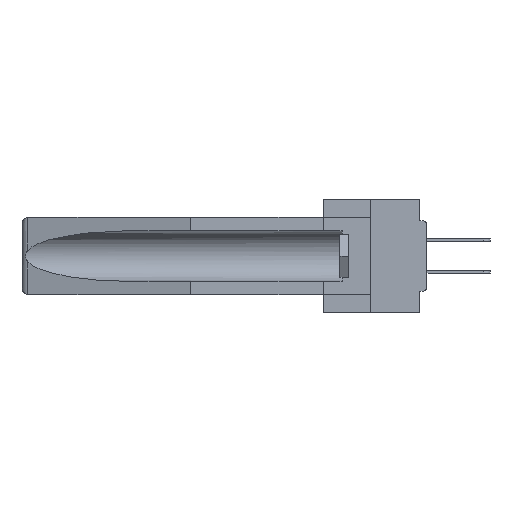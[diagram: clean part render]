
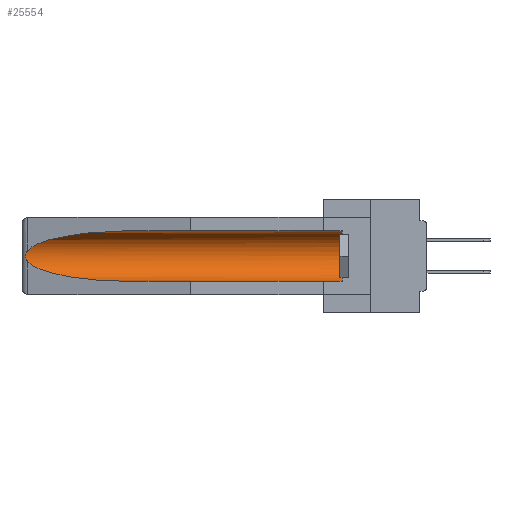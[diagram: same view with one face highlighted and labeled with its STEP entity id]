
A CAD part, left-side view. The second image highlights one B-rep face of the part: STEP entity #25554.
In plain terms, the highlighted cylindrical face has radius 2.857 mm (diameter 5.715 mm), a partial arc.
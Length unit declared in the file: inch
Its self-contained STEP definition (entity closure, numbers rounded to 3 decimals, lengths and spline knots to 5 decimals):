
#349 = EDGE_CURVE ( 'NONE', #12843, #17895, #983, .T. ) ;
#506 = VERTEX_POINT ( 'NONE', #14786 ) ;
#983 =( BOUNDED_CURVE ( )  B_SPLINE_CURVE ( 3, ( #24447, #27246, #11314, #16499 ),
 .UNSPECIFIED., .F., .F. ) 
 B_SPLINE_CURVE_WITH_KNOTS ( ( 4, 4 ),
 ( 4.71239, 6.08839 ),
 .UNSPECIFIED. ) 
 CURVE ( )  GEOMETRIC_REPRESENTATION_ITEM ( )  RATIONAL_B_SPLINE_CURVE ( ( 1., 0.848, 0.848, 1. ) ) 
 REPRESENTATION_ITEM ( '' )  );
#1634 = VECTOR ( 'NONE', #4664, 39.37008 ) ;
#1759 = AXIS2_PLACEMENT_3D ( 'NONE', #3451, #17104, #19829 ) ;
#2175 = CIRCLE ( 'NONE', #19865, 0.1125 ) ;
#3451 = CARTESIAN_POINT ( 'NONE',  ( 0.155, -0.30754, -0.1715 ) ) ;
#3897 = VECTOR ( 'NONE', #30911, 39.37008 ) ;
#4554 = CARTESIAN_POINT ( 'NONE',  ( 0.155, -0.30754, -0.284 ) ) ;
#4664 = DIRECTION ( 'NONE',  ( 0., 1., 0. ) ) ;
#4744 = DIRECTION ( 'NONE',  ( 0., 0., 1. ) ) ;
#4749 = VERTEX_POINT ( 'NONE', #17183 ) ;
#5481 = CARTESIAN_POINT ( 'NONE',  ( 0.21114, 1.30732, -0.284 ) ) ;
#5918 = ORIENTED_EDGE ( 'NONE', *, *, #8402, .T. ) ;
#6182 = CARTESIAN_POINT ( 'NONE',  ( 0.2673, 1.5327, -0.16383 ) ) ;
#6440 = CARTESIAN_POINT ( 'NONE',  ( 0.26597, 1.5296, -0.19026 ) ) ;
#8402 = EDGE_CURVE ( 'NONE', #28125, #16788, #17603, .T. ) ;
#8495 = CARTESIAN_POINT ( 'NONE',  ( 0.26537, 1.52718, -0.19328 ) ) ;
#9487 = CARTESIAN_POINT ( 'NONE',  ( 0.26537, 1.52718, -0.19328 ) ) ;
#11211 = CARTESIAN_POINT ( 'NONE',  ( 0.2675, 1.53308, -0.16763 ) ) ;
#11274 = ORIENTED_EDGE ( 'NONE', *, *, #27822, .T. ) ;
#11314 = CARTESIAN_POINT ( 'NONE',  ( 0.25451, 1.48313, -0.09465 ) ) ;
#11803 = EDGE_CURVE ( 'NONE', #506, #16788, #28668, .T. ) ;
#11893 = B_SPLINE_CURVE_WITH_KNOTS ( 'NONE', 3,
 ( #27144, #13857, #22145, #6182, #11211, #14679, #19572, #33063, #6440, #27606 ),
 .UNSPECIFIED., .F., .F.,
 ( 4, 2, 2, 2, 4 ),
 ( 0., 0.00029, 0.00058, 0.00087, 0.00117 ),
 .UNSPECIFIED. ) ;
#12843 = VERTEX_POINT ( 'NONE', #13403 ) ;
#13199 = ORIENTED_EDGE ( 'NONE', *, *, #349, .T. ) ;
#13403 = CARTESIAN_POINT ( 'NONE',  ( 0.155, 1.07973, -0.059 ) ) ;
#13857 = CARTESIAN_POINT ( 'NONE',  ( 0.26597, 1.52961, -0.15275 ) ) ;
#13952 = CARTESIAN_POINT ( 'NONE',  ( 0.25451, 1.48313, -0.24835 ) ) ;
#14679 = CARTESIAN_POINT ( 'NONE',  ( 0.2675, 1.53308, -0.17534 ) ) ;
#14732 = ORIENTED_EDGE ( 'NONE', *, *, #21017, .T. ) ;
#14786 = CARTESIAN_POINT ( 'NONE',  ( 0.155, 0.126, -0.284 ) ) ;
#15538 = CARTESIAN_POINT ( 'NONE',  ( 0.155, 0.126, -0.1715 ) ) ;
#16072 = CARTESIAN_POINT ( 'NONE',  ( 0.26537, 1.52718, -0.14972 ) ) ;
#16499 = CARTESIAN_POINT ( 'NONE',  ( 0.26537, 1.52718, -0.14972 ) ) ;
#16788 = VERTEX_POINT ( 'NONE', #32964 ) ;
#17104 = DIRECTION ( 'NONE',  ( 0., 1., 0. ) ) ;
#17183 = CARTESIAN_POINT ( 'NONE',  ( 0.155, 0.126, -0.059 ) ) ;
#17603 =( BOUNDED_CURVE ( )  B_SPLINE_CURVE ( 3, ( #8495, #13952, #5481, #26779 ),
 .UNSPECIFIED., .F., .F. ) 
 B_SPLINE_CURVE_WITH_KNOTS ( ( 4, 4 ),
 ( 0.1948, 1.5708 ),
 .UNSPECIFIED. ) 
 CURVE ( )  GEOMETRIC_REPRESENTATION_ITEM ( )  RATIONAL_B_SPLINE_CURVE ( ( 1., 0.848, 0.848, 1. ) ) 
 REPRESENTATION_ITEM ( '' )  );
#17895 = VERTEX_POINT ( 'NONE', #16072 ) ;
#19572 = CARTESIAN_POINT ( 'NONE',  ( 0.2673, 1.53269, -0.17917 ) ) ;
#19829 = DIRECTION ( 'NONE',  ( 0., 0., 1. ) ) ;
#19865 = AXIS2_PLACEMENT_3D ( 'NONE', #15538, #31248, #4744 ) ;
#21017 = EDGE_CURVE ( 'NONE', #17895, #28125, #11893, .T. ) ;
#22145 = CARTESIAN_POINT ( 'NONE',  ( 0.26654, 1.53092, -0.15636 ) ) ;
#22932 = CARTESIAN_POINT ( 'NONE',  ( 0.155, -0.30754, -0.059 ) ) ;
#24447 = CARTESIAN_POINT ( 'NONE',  ( 0.155, 1.07973, -0.059 ) ) ;
#25554 = ADVANCED_FACE ( 'NONE', ( #28925 ), #28104, .F. ) ;
#25887 = ORIENTED_EDGE ( 'NONE', *, *, #11803, .F. ) ;
#26641 = ORIENTED_EDGE ( 'NONE', *, *, #33832, .T. ) ;
#26779 = CARTESIAN_POINT ( 'NONE',  ( 0.155, 1.07973, -0.284 ) ) ;
#27144 = CARTESIAN_POINT ( 'NONE',  ( 0.26537, 1.52718, -0.14972 ) ) ;
#27246 = CARTESIAN_POINT ( 'NONE',  ( 0.21114, 1.30732, -0.059 ) ) ;
#27606 = CARTESIAN_POINT ( 'NONE',  ( 0.26537, 1.52718, -0.19328 ) ) ;
#27822 = EDGE_CURVE ( 'NONE', #506, #4749, #2175, .T. ) ;
#28104 = CYLINDRICAL_SURFACE ( 'NONE', #1759, 0.1125 ) ;
#28125 = VERTEX_POINT ( 'NONE', #9487 ) ;
#28668 = LINE ( 'NONE', #4554, #1634 ) ;
#28925 = FACE_OUTER_BOUND ( 'NONE', #30764, .T. ) ;
#30764 = EDGE_LOOP ( 'NONE', ( #13199, #14732, #5918, #25887, #11274, #26641 ) ) ;
#30911 = DIRECTION ( 'NONE',  ( 0., 1., 0. ) ) ;
#31248 = DIRECTION ( 'NONE',  ( 0., -1., 0. ) ) ;
#32156 = LINE ( 'NONE', #22932, #3897 ) ;
#32964 = CARTESIAN_POINT ( 'NONE',  ( 0.155, 1.07973, -0.284 ) ) ;
#33063 = CARTESIAN_POINT ( 'NONE',  ( 0.26655, 1.53094, -0.18657 ) ) ;
#33832 = EDGE_CURVE ( 'NONE', #4749, #12843, #32156, .T. ) ;
